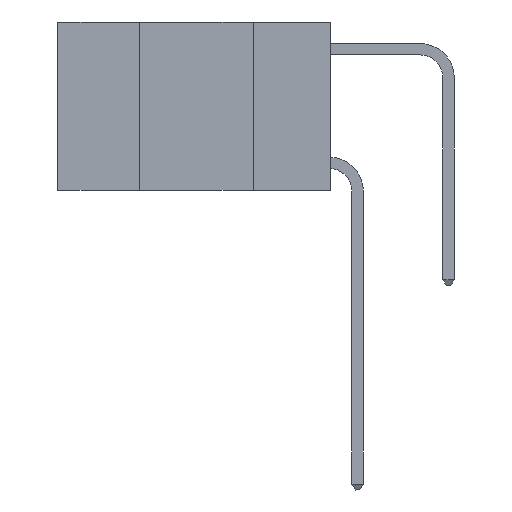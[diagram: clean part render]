
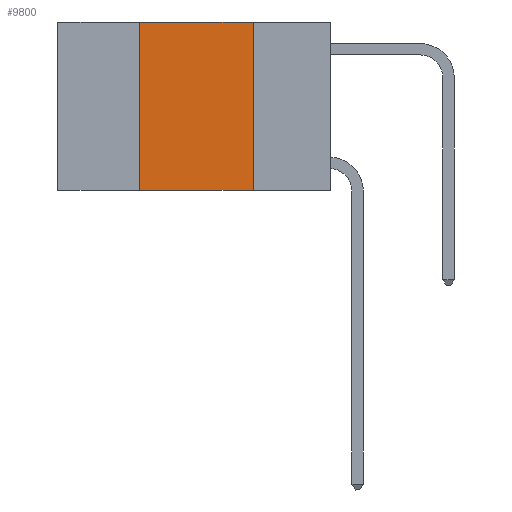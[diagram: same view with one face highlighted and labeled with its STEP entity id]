
A CAD part, left-side view. The second image highlights one B-rep face of the part: STEP entity #9800.
In plain terms, the highlighted planar face has unit normal (-1, 0, 0).
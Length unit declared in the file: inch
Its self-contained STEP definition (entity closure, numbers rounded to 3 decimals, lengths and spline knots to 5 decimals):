
#243 = PLANE ( 'NONE',  #638 ) ;
#638 = AXIS2_PLACEMENT_3D ( 'NONE', #3487, #11492, #6223 ) ;
#1124 = EDGE_CURVE ( 'NONE', #6151, #7925, #11787, .T. ) ;
#2226 = FACE_OUTER_BOUND ( 'NONE', #5187, .T. ) ;
#2392 = LINE ( 'NONE', #3281, #4648 ) ;
#2475 = EDGE_CURVE ( 'NONE', #3908, #7925, #2392, .T. ) ;
#3147 = CARTESIAN_POINT ( 'NONE',  ( 0., 0.17, 0. ) ) ;
#3281 = CARTESIAN_POINT ( 'NONE',  ( 0., 0.17, 0. ) ) ;
#3487 = CARTESIAN_POINT ( 'NONE',  ( 0., 0.6, 0. ) ) ;
#3908 = VERTEX_POINT ( 'NONE', #3147 ) ;
#3913 = VERTEX_POINT ( 'NONE', #10342 ) ;
#4648 = VECTOR ( 'NONE', #5304, 39.37008 ) ;
#4783 = ORIENTED_EDGE ( 'NONE', *, *, #9505, .F. ) ;
#5009 = EDGE_CURVE ( 'NONE', #3913, #3908, #9297, .T. ) ;
#5097 = CARTESIAN_POINT ( 'NONE',  ( 0., 0.42, 0. ) ) ;
#5187 = EDGE_LOOP ( 'NONE', ( #7215, #6138, #4783, #6426 ) ) ;
#5293 = DIRECTION ( 'NONE',  ( 0., -1., 0. ) ) ;
#5304 = DIRECTION ( 'NONE',  ( 0., 0., -1. ) ) ;
#5443 = DIRECTION ( 'NONE',  ( 0., -1., 0. ) ) ;
#5974 = VECTOR ( 'NONE', #5443, 39.37008 ) ;
#6138 = ORIENTED_EDGE ( 'NONE', *, *, #5009, .F. ) ;
#6151 = VERTEX_POINT ( 'NONE', #10987 ) ;
#6223 = DIRECTION ( 'NONE',  ( 0., 0., -1. ) ) ;
#6426 = ORIENTED_EDGE ( 'NONE', *, *, #1124, .T. ) ;
#7103 = VECTOR ( 'NONE', #5293, 39.37008 ) ;
#7215 = ORIENTED_EDGE ( 'NONE', *, *, #2475, .F. ) ;
#7925 = VERTEX_POINT ( 'NONE', #11161 ) ;
#9116 = LINE ( 'NONE', #5097, #11391 ) ;
#9297 = LINE ( 'NONE', #9862, #5974 ) ;
#9505 = EDGE_CURVE ( 'NONE', #6151, #3913, #9116, .T. ) ;
#9800 = ADVANCED_FACE ( 'NONE', ( #2226 ), #243, .F. ) ;
#9862 = CARTESIAN_POINT ( 'NONE',  ( 0., 0.6, 0. ) ) ;
#10342 = CARTESIAN_POINT ( 'NONE',  ( 0., 0.42, 0. ) ) ;
#10987 = CARTESIAN_POINT ( 'NONE',  ( 0., 0.42, -0.37 ) ) ;
#11161 = CARTESIAN_POINT ( 'NONE',  ( 0., 0.17, -0.37 ) ) ;
#11249 = DIRECTION ( 'NONE',  ( 0., 0., 1. ) ) ;
#11391 = VECTOR ( 'NONE', #11249, 39.37008 ) ;
#11492 = DIRECTION ( 'NONE',  ( 1., 0., 0. ) ) ;
#11787 = LINE ( 'NONE', #12062, #7103 ) ;
#12062 = CARTESIAN_POINT ( 'NONE',  ( 0., 0.6, -0.37 ) ) ;
